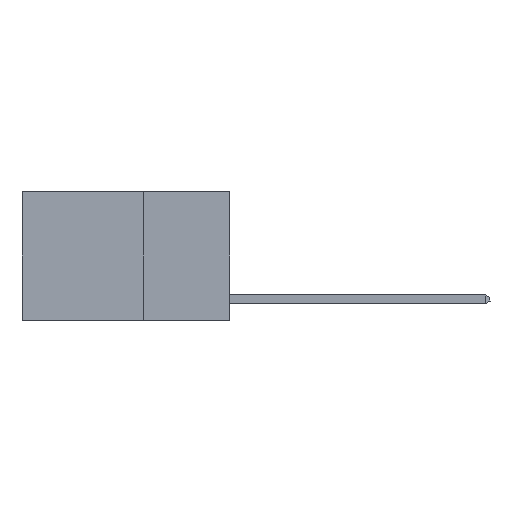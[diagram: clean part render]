
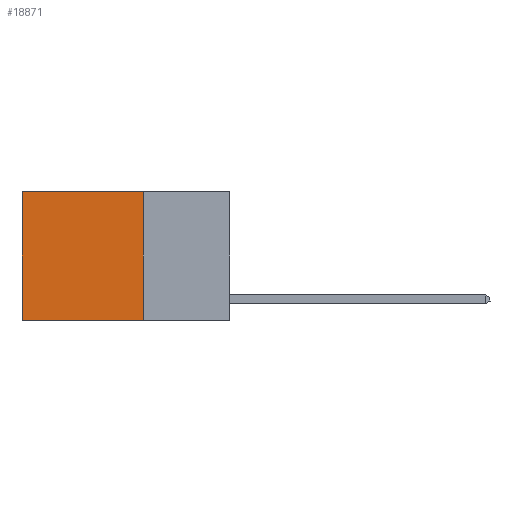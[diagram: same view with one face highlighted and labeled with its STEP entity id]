
A CAD part, left-side view. The second image highlights one B-rep face of the part: STEP entity #18871.
In plain terms, the highlighted planar face has unit normal (-1, 0, 0).
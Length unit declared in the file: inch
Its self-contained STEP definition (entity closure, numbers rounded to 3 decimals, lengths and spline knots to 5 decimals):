
#398 = AXIS2_PLACEMENT_3D ( 'NONE', #7521, #4454, #15273 ) ;
#931 = ORIENTED_EDGE ( 'NONE', *, *, #8082, .T. ) ;
#1124 = DIRECTION ( 'NONE',  ( 0., 0., -1. ) ) ;
#1524 = CARTESIAN_POINT ( 'NONE',  ( 0.2625, 0.6, 0. ) ) ;
#2290 = EDGE_CURVE ( 'NONE', #16153, #14477, #14606, .T. ) ;
#2616 = CARTESIAN_POINT ( 'NONE',  ( 0.2625, 0.6, 0. ) ) ;
#2917 = CARTESIAN_POINT ( 'NONE',  ( 0.2625, 0.25, -0.37 ) ) ;
#2949 = CARTESIAN_POINT ( 'NONE',  ( 0.2625, 0.25, 0. ) ) ;
#3092 = ORIENTED_EDGE ( 'NONE', *, *, #2290, .T. ) ;
#3235 = VECTOR ( 'NONE', #4507, 39.37008 ) ;
#3427 = LINE ( 'NONE', #18053, #13345 ) ;
#4283 = CARTESIAN_POINT ( 'NONE',  ( 0.2625, 0.25, 0. ) ) ;
#4353 = DIRECTION ( 'NONE',  ( 0., 0., -1. ) ) ;
#4454 = DIRECTION ( 'NONE',  ( 1., 0., 0. ) ) ;
#4507 = DIRECTION ( 'NONE',  ( 0., 1., 0. ) ) ;
#5104 = EDGE_LOOP ( 'NONE', ( #931, #13447, #6293, #3092 ) ) ;
#5397 = EDGE_CURVE ( 'NONE', #16153, #7047, #13994, .T. ) ;
#5865 = DIRECTION ( 'NONE',  ( 0., 1., 0. ) ) ;
#6293 = ORIENTED_EDGE ( 'NONE', *, *, #5397, .F. ) ;
#6569 = FACE_OUTER_BOUND ( 'NONE', #5104, .T. ) ;
#7047 = VERTEX_POINT ( 'NONE', #2917 ) ;
#7521 = CARTESIAN_POINT ( 'NONE',  ( 0.2625, 0.25, 0. ) ) ;
#8082 = EDGE_CURVE ( 'NONE', #14477, #18241, #10414, .T. ) ;
#9917 = VECTOR ( 'NONE', #4353, 39.37008 ) ;
#10414 = LINE ( 'NONE', #2616, #18086 ) ;
#10635 = PLANE ( 'NONE',  #398 ) ;
#12438 = EDGE_CURVE ( 'NONE', #7047, #18241, #3427, .T. ) ;
#13345 = VECTOR ( 'NONE', #5865, 39.37008 ) ;
#13447 = ORIENTED_EDGE ( 'NONE', *, *, #12438, .F. ) ;
#13994 = LINE ( 'NONE', #4283, #9917 ) ;
#14477 = VERTEX_POINT ( 'NONE', #1524 ) ;
#14606 = LINE ( 'NONE', #2949, #3235 ) ;
#15273 = DIRECTION ( 'NONE',  ( 0., 0., -1. ) ) ;
#16110 = CARTESIAN_POINT ( 'NONE',  ( 0.2625, 0.25, 0. ) ) ;
#16153 = VERTEX_POINT ( 'NONE', #16110 ) ;
#16780 = CARTESIAN_POINT ( 'NONE',  ( 0.2625, 0.6, -0.37 ) ) ;
#18053 = CARTESIAN_POINT ( 'NONE',  ( 0.2625, 0.25, -0.37 ) ) ;
#18086 = VECTOR ( 'NONE', #1124, 39.37008 ) ;
#18241 = VERTEX_POINT ( 'NONE', #16780 ) ;
#18871 = ADVANCED_FACE ( 'NONE', ( #6569 ), #10635, .F. ) ;
